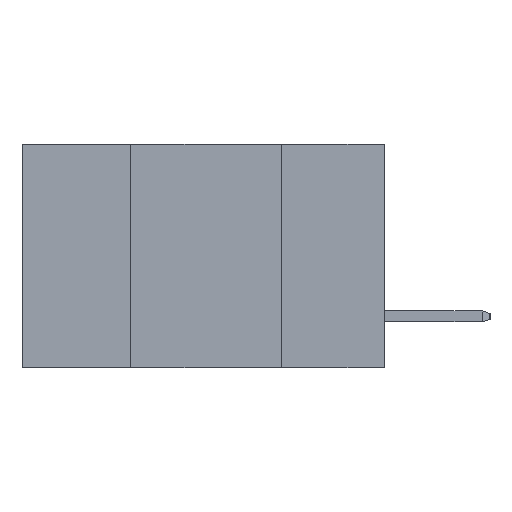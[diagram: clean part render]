
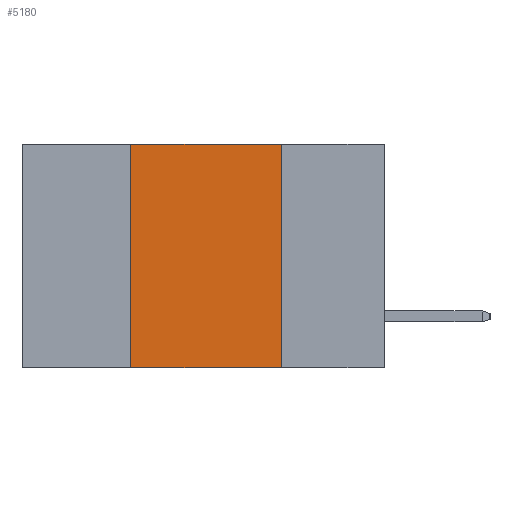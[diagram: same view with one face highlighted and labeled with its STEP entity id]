
A CAD part, left-side view. The second image highlights one B-rep face of the part: STEP entity #5180.
In plain terms, the highlighted planar face has unit normal (-1, 0, 0).
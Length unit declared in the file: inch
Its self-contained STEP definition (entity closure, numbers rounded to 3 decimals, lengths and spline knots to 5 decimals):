
#255 = AXIS2_PLACEMENT_3D ( 'NONE', #8169, #8560, #4745 ) ;
#398 = CARTESIAN_POINT ( 'NONE',  ( 0., 0.6, 0. ) ) ;
#1137 = DIRECTION ( 'NONE',  ( 0., -1., 0. ) ) ;
#1319 = EDGE_LOOP ( 'NONE', ( #8984, #1996, #6376, #5847 ) ) ;
#1948 = VECTOR ( 'NONE', #1137, 39.37008 ) ;
#1996 = ORIENTED_EDGE ( 'NONE', *, *, #8120, .F. ) ;
#2001 = VERTEX_POINT ( 'NONE', #5574 ) ;
#2414 = EDGE_CURVE ( 'NONE', #2001, #5007, #4810, .T. ) ;
#2650 = CARTESIAN_POINT ( 'NONE',  ( 0., 0.42, -0.37 ) ) ;
#2676 = LINE ( 'NONE', #8387, #4543 ) ;
#3037 = FACE_OUTER_BOUND ( 'NONE', #1319, .T. ) ;
#3229 = CARTESIAN_POINT ( 'NONE',  ( 0., 0.17, 0. ) ) ;
#4265 = VERTEX_POINT ( 'NONE', #5373 ) ;
#4543 = VECTOR ( 'NONE', #8493, 39.37008 ) ;
#4625 = DIRECTION ( 'NONE',  ( 0., -1., 0. ) ) ;
#4711 = CARTESIAN_POINT ( 'NONE',  ( 0., 0.6, -0.37 ) ) ;
#4745 = DIRECTION ( 'NONE',  ( 0., 0., -1. ) ) ;
#4810 = LINE ( 'NONE', #2650, #6428 ) ;
#4981 = VERTEX_POINT ( 'NONE', #3229 ) ;
#5007 = VERTEX_POINT ( 'NONE', #6018 ) ;
#5180 = ADVANCED_FACE ( 'NONE', ( #3037 ), #8939, .F. ) ;
#5352 = EDGE_CURVE ( 'NONE', #2001, #4265, #8983, .T. ) ;
#5373 = CARTESIAN_POINT ( 'NONE',  ( 0., 0.17, -0.37 ) ) ;
#5453 = VECTOR ( 'NONE', #4625, 39.37008 ) ;
#5574 = CARTESIAN_POINT ( 'NONE',  ( 0., 0.42, -0.37 ) ) ;
#5847 = ORIENTED_EDGE ( 'NONE', *, *, #5352, .T. ) ;
#6018 = CARTESIAN_POINT ( 'NONE',  ( 0., 0.42, 0. ) ) ;
#6331 = EDGE_CURVE ( 'NONE', #4981, #4265, #2676, .T. ) ;
#6376 = ORIENTED_EDGE ( 'NONE', *, *, #2414, .F. ) ;
#6428 = VECTOR ( 'NONE', #8320, 39.37008 ) ;
#7487 = LINE ( 'NONE', #398, #1948 ) ;
#8120 = EDGE_CURVE ( 'NONE', #5007, #4981, #7487, .T. ) ;
#8169 = CARTESIAN_POINT ( 'NONE',  ( 0., 0.6, 0. ) ) ;
#8320 = DIRECTION ( 'NONE',  ( 0., 0., 1. ) ) ;
#8387 = CARTESIAN_POINT ( 'NONE',  ( 0., 0.17, -0.37 ) ) ;
#8493 = DIRECTION ( 'NONE',  ( 0., 0., -1. ) ) ;
#8560 = DIRECTION ( 'NONE',  ( 1., 0., 0. ) ) ;
#8939 = PLANE ( 'NONE',  #255 ) ;
#8983 = LINE ( 'NONE', #4711, #5453 ) ;
#8984 = ORIENTED_EDGE ( 'NONE', *, *, #6331, .F. ) ;
